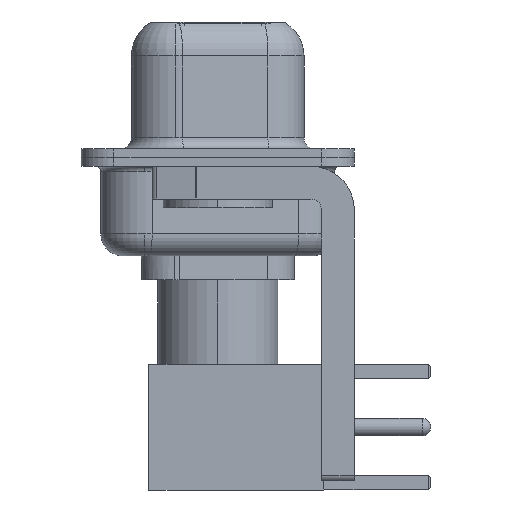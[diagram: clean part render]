
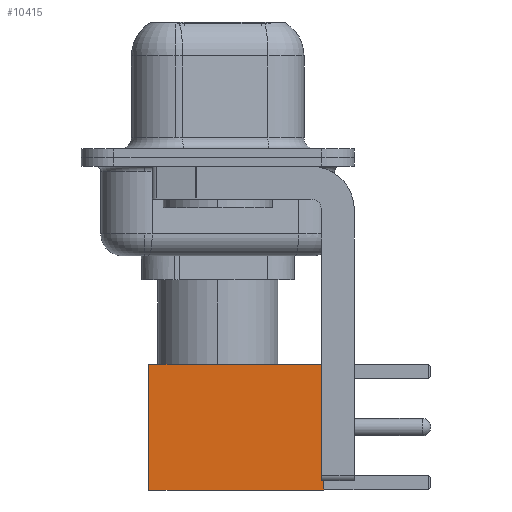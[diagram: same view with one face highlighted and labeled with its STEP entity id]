
A CAD part, left-side view. The second image highlights one B-rep face of the part: STEP entity #10415.
In plain terms, the highlighted face is planar.
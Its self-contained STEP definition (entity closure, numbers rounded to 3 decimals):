
#278 = VERTEX_POINT ( 'NONE', #11546 ) ;
#950 = VERTEX_POINT ( 'NONE', #11611 ) ;
#1260 = EDGE_LOOP ( 'NONE', ( #13165, #11038, #12151, #15324 ) ) ;
#2651 = DIRECTION ( 'NONE',  ( 0., 1., 0. ) ) ;
#2674 = CARTESIAN_POINT ( 'NONE',  ( 2.875, 2.875, 0. ) ) ;
#3662 = CARTESIAN_POINT ( 'NONE',  ( 2.875, 2.875, 0. ) ) ;
#3827 = DIRECTION ( 'NONE',  ( -1., 0., 0. ) ) ;
#3968 = CARTESIAN_POINT ( 'NONE',  ( 0., 2.875, 8. ) ) ;
#4342 = CARTESIAN_POINT ( 'NONE',  ( -2.875, 2.875, 8. ) ) ;
#4457 = EDGE_CURVE ( 'NONE', #13195, #950, #15498, .T. ) ;
#4879 = AXIS2_PLACEMENT_3D ( 'NONE', #3662, #2651, #8936 ) ;
#4930 = CARTESIAN_POINT ( 'NONE',  ( 2.875, 2.875, 0. ) ) ;
#5023 = FACE_OUTER_BOUND ( 'NONE', #1260, .T. ) ;
#5164 = LINE ( 'NONE', #3968, #14651 ) ;
#5367 = EDGE_CURVE ( 'NONE', #13206, #950, #6684, .T. ) ;
#6684 = LINE ( 'NONE', #14482, #16177 ) ;
#7696 = EDGE_CURVE ( 'NONE', #278, #13206, #5164, .T. ) ;
#7833 = LINE ( 'NONE', #4930, #13162 ) ;
#8854 = PLANE ( 'NONE',  #4879 ) ;
#8936 = DIRECTION ( 'NONE',  ( 0., 0., 1. ) ) ;
#9042 = DIRECTION ( 'NONE',  ( 0., 0., -1. ) ) ;
#9423 = VECTOR ( 'NONE', #3827, 1000. ) ;
#10147 = DIRECTION ( 'NONE',  ( 0., 0., -1. ) ) ;
#10415 = ADVANCED_FACE ( 'NONE', ( #5023 ), #8854, .T. ) ;
#11038 = ORIENTED_EDGE ( 'NONE', *, *, #4457, .T. ) ;
#11399 = CARTESIAN_POINT ( 'NONE',  ( 0., 2.875, 0. ) ) ;
#11546 = CARTESIAN_POINT ( 'NONE',  ( 2.875, 2.875, 8. ) ) ;
#11611 = CARTESIAN_POINT ( 'NONE',  ( -2.875, 2.875, 0. ) ) ;
#12151 = ORIENTED_EDGE ( 'NONE', *, *, #5367, .F. ) ;
#12905 = DIRECTION ( 'NONE',  ( -1., 0., 0. ) ) ;
#13162 = VECTOR ( 'NONE', #10147, 1000. ) ;
#13165 = ORIENTED_EDGE ( 'NONE', *, *, #16619, .T. ) ;
#13195 = VERTEX_POINT ( 'NONE', #2674 ) ;
#13206 = VERTEX_POINT ( 'NONE', #4342 ) ;
#14482 = CARTESIAN_POINT ( 'NONE',  ( -2.875, 2.875, 0. ) ) ;
#14651 = VECTOR ( 'NONE', #12905, 1000. ) ;
#15324 = ORIENTED_EDGE ( 'NONE', *, *, #7696, .F. ) ;
#15498 = LINE ( 'NONE', #11399, #9423 ) ;
#16177 = VECTOR ( 'NONE', #9042, 1000. ) ;
#16619 = EDGE_CURVE ( 'NONE', #278, #13195, #7833, .T. ) ;
